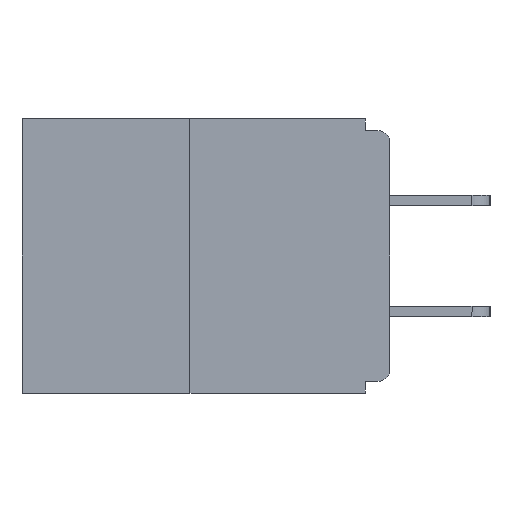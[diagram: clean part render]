
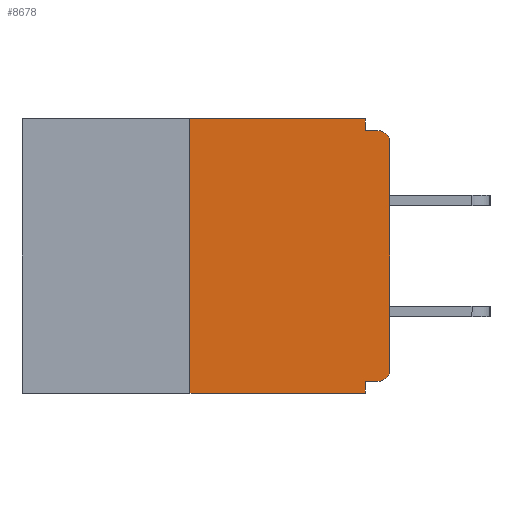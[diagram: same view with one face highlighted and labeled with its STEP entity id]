
A CAD part, left-side view. The second image highlights one B-rep face of the part: STEP entity #8678.
In plain terms, the highlighted planar face has unit normal (-1, 0, 0).
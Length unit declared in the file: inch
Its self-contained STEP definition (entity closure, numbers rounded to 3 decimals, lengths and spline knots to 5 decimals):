
#16 = ORIENTED_EDGE ( 'NONE', *, *, #22209, .T. ) ;
#254 = CARTESIAN_POINT ( 'NONE',  ( 0., 0.031, -0.328 ) ) ;
#372 = CARTESIAN_POINT ( 'NONE',  ( 0., 0., 0. ) ) ;
#455 = LINE ( 'NONE', #24782, #4114 ) ;
#656 = ORIENTED_EDGE ( 'NONE', *, *, #3587, .T. ) ;
#993 = EDGE_CURVE ( 'NONE', #1116, #14769, #455, .T. ) ;
#1116 = VERTEX_POINT ( 'NONE', #23750 ) ;
#1211 = DIRECTION ( 'NONE',  ( 0., 0., -1. ) ) ;
#1274 = LINE ( 'NONE', #6727, #1541 ) ;
#1541 = VECTOR ( 'NONE', #4590, 39.37008 ) ;
#2590 = DIRECTION ( 'NONE',  ( 1., 0., 0. ) ) ;
#2661 = VECTOR ( 'NONE', #25285, 39.37008 ) ;
#2980 = CARTESIAN_POINT ( 'NONE',  ( 0., 0.015, -0.313 ) ) ;
#2988 = AXIS2_PLACEMENT_3D ( 'NONE', #16330, #2590, #16082 ) ;
#3587 = EDGE_CURVE ( 'NONE', #17428, #21058, #12883, .T. ) ;
#3765 = CARTESIAN_POINT ( 'NONE',  ( 0., 0.031, 0. ) ) ;
#3800 = DIRECTION ( 'NONE',  ( 0., 0., -1. ) ) ;
#3939 = CARTESIAN_POINT ( 'NONE',  ( 0., 0.031, -0.015 ) ) ;
#4067 = EDGE_LOOP ( 'NONE', ( #9620, #7439, #19907, #8168, #21882, #656, #25349, #16, #14035, #14601 ) ) ;
#4114 = VECTOR ( 'NONE', #12870, 39.37008 ) ;
#4155 = VECTOR ( 'NONE', #17847, 39.37008 ) ;
#4236 = AXIS2_PLACEMENT_3D ( 'NONE', #17560, #5967, #3800 ) ;
#4590 = DIRECTION ( 'NONE',  ( 0., 0., -1. ) ) ;
#4836 = VERTEX_POINT ( 'NONE', #23437 ) ;
#5129 = LINE ( 'NONE', #17128, #2661 ) ;
#5967 = DIRECTION ( 'NONE',  ( -1., 0., 0. ) ) ;
#6727 = CARTESIAN_POINT ( 'NONE',  ( 0., 0.031, -0.343 ) ) ;
#6910 = LINE ( 'NONE', #23679, #4155 ) ;
#6948 = VERTEX_POINT ( 'NONE', #11167 ) ;
#7002 = EDGE_CURVE ( 'NONE', #17428, #18418, #15458, .T. ) ;
#7439 = ORIENTED_EDGE ( 'NONE', *, *, #22099, .F. ) ;
#8168 = ORIENTED_EDGE ( 'NONE', *, *, #13636, .F. ) ;
#8678 = ADVANCED_FACE ( 'NONE', ( #18408 ), #19947, .F. ) ;
#9620 = ORIENTED_EDGE ( 'NONE', *, *, #16383, .F. ) ;
#10002 = LINE ( 'NONE', #17839, #13719 ) ;
#11167 = CARTESIAN_POINT ( 'NONE',  ( 0., 0.015, -0.015 ) ) ;
#11841 = DIRECTION ( 'NONE',  ( 0., 1., 0. ) ) ;
#12715 = EDGE_CURVE ( 'NONE', #21058, #4836, #22136, .T. ) ;
#12870 = DIRECTION ( 'NONE',  ( 0., -1., 0. ) ) ;
#12883 = CIRCLE ( 'NONE', #14450, 0.015 ) ;
#13578 = CARTESIAN_POINT ( 'NONE',  ( 0., 0., -0.328 ) ) ;
#13636 = EDGE_CURVE ( 'NONE', #18418, #14769, #1274, .T. ) ;
#13719 = VECTOR ( 'NONE', #24003, 39.37008 ) ;
#14035 = ORIENTED_EDGE ( 'NONE', *, *, #23292, .F. ) ;
#14104 = DIRECTION ( 'NONE',  ( 0., 0., 1. ) ) ;
#14243 = LINE ( 'NONE', #16868, #25295 ) ;
#14450 = AXIS2_PLACEMENT_3D ( 'NONE', #2980, #24883, #1211 ) ;
#14601 = ORIENTED_EDGE ( 'NONE', *, *, #24460, .F. ) ;
#14769 = VERTEX_POINT ( 'NONE', #21864 ) ;
#15458 = LINE ( 'NONE', #13578, #17576 ) ;
#16082 = DIRECTION ( 'NONE',  ( 0., 0., -1. ) ) ;
#16330 = CARTESIAN_POINT ( 'NONE',  ( 0., 0.46, 0. ) ) ;
#16383 = EDGE_CURVE ( 'NONE', #22471, #25305, #6910, .T. ) ;
#16609 = DIRECTION ( 'NONE',  ( 0., 0., -1. ) ) ;
#16868 = CARTESIAN_POINT ( 'NONE',  ( 0., 0.031, 0. ) ) ;
#17128 = CARTESIAN_POINT ( 'NONE',  ( 0., 0.25, 0. ) ) ;
#17428 = VERTEX_POINT ( 'NONE', #24596 ) ;
#17544 = VECTOR ( 'NONE', #14104, 39.37008 ) ;
#17560 = CARTESIAN_POINT ( 'NONE',  ( 0., 0.015, -0.03 ) ) ;
#17576 = VECTOR ( 'NONE', #11841, 39.37008 ) ;
#17839 = CARTESIAN_POINT ( 'NONE',  ( 0., 0., -0.015 ) ) ;
#17847 = DIRECTION ( 'NONE',  ( 0., -1., 0. ) ) ;
#18408 = FACE_OUTER_BOUND ( 'NONE', #4067, .T. ) ;
#18418 = VERTEX_POINT ( 'NONE', #254 ) ;
#19290 = CIRCLE ( 'NONE', #4236, 0.015 ) ;
#19426 = VERTEX_POINT ( 'NONE', #3939 ) ;
#19907 = ORIENTED_EDGE ( 'NONE', *, *, #993, .T. ) ;
#19947 = PLANE ( 'NONE',  #2988 ) ;
#20456 = CARTESIAN_POINT ( 'NONE',  ( 0., 0.25, 0. ) ) ;
#21058 = VERTEX_POINT ( 'NONE', #21239 ) ;
#21239 = CARTESIAN_POINT ( 'NONE',  ( 0., 0., -0.313 ) ) ;
#21864 = CARTESIAN_POINT ( 'NONE',  ( 0., 0.031, -0.343 ) ) ;
#21882 = ORIENTED_EDGE ( 'NONE', *, *, #7002, .F. ) ;
#22099 = EDGE_CURVE ( 'NONE', #1116, #22471, #5129, .T. ) ;
#22136 = LINE ( 'NONE', #372, #17544 ) ;
#22209 = EDGE_CURVE ( 'NONE', #4836, #6948, #19290, .T. ) ;
#22471 = VERTEX_POINT ( 'NONE', #20456 ) ;
#23292 = EDGE_CURVE ( 'NONE', #19426, #6948, #10002, .T. ) ;
#23437 = CARTESIAN_POINT ( 'NONE',  ( 0., 0., -0.03 ) ) ;
#23679 = CARTESIAN_POINT ( 'NONE',  ( 0., 0.46, 0. ) ) ;
#23750 = CARTESIAN_POINT ( 'NONE',  ( 0., 0.25, -0.343 ) ) ;
#24003 = DIRECTION ( 'NONE',  ( 0., -1., 0. ) ) ;
#24460 = EDGE_CURVE ( 'NONE', #25305, #19426, #14243, .T. ) ;
#24596 = CARTESIAN_POINT ( 'NONE',  ( 0., 0.015, -0.328 ) ) ;
#24782 = CARTESIAN_POINT ( 'NONE',  ( 0., 0.46, -0.343 ) ) ;
#24883 = DIRECTION ( 'NONE',  ( -1., 0., 0. ) ) ;
#25285 = DIRECTION ( 'NONE',  ( 0., 0., 1. ) ) ;
#25295 = VECTOR ( 'NONE', #16609, 39.37008 ) ;
#25305 = VERTEX_POINT ( 'NONE', #3765 ) ;
#25349 = ORIENTED_EDGE ( 'NONE', *, *, #12715, .T. ) ;
